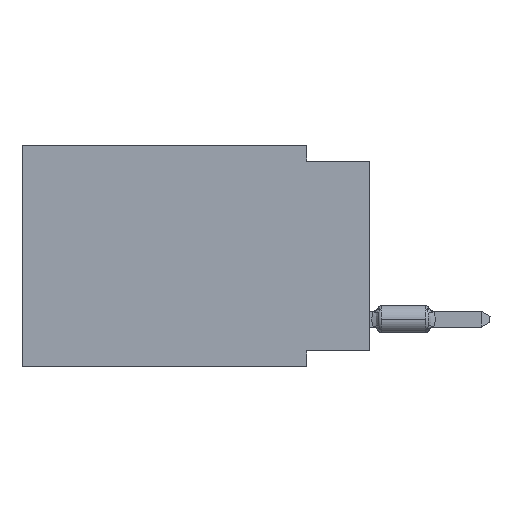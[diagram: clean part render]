
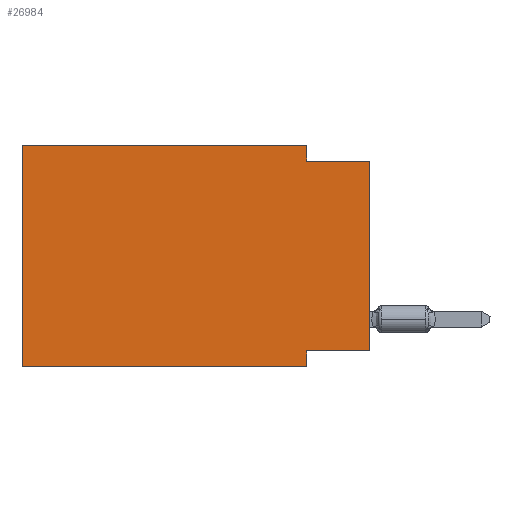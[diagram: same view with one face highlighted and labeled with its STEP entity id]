
A CAD part, left-side view. The second image highlights one B-rep face of the part: STEP entity #26984.
In plain terms, the highlighted planar face has unit normal (-1, 0, 0).
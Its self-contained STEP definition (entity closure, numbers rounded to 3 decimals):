
#285 = CARTESIAN_POINT ( 'NONE',  ( 0., 0., 0. ) ) ;
#792 = EDGE_CURVE ( 'NONE', #8059, #13492, #8434, .T. ) ;
#1193 = CARTESIAN_POINT ( 'NONE',  ( 0., 13.97, 0. ) ) ;
#1376 = LINE ( 'NONE', #13339, #2917 ) ;
#1518 = DIRECTION ( 'NONE',  ( 0., 0., -1. ) ) ;
#1552 = EDGE_CURVE ( 'NONE', #6276, #4184, #1376, .T. ) ;
#1612 = VECTOR ( 'NONE', #5593, 1000. ) ;
#1781 = ORIENTED_EDGE ( 'NONE', *, *, #23524, .F. ) ;
#2917 = VECTOR ( 'NONE', #1518, 1000. ) ;
#2962 = CARTESIAN_POINT ( 'NONE',  ( 0., 13.97, 0. ) ) ;
#3101 = ORIENTED_EDGE ( 'NONE', *, *, #22007, .F. ) ;
#3314 = VECTOR ( 'NONE', #18059, 1000. ) ;
#3389 = VERTEX_POINT ( 'NONE', #10796 ) ;
#4184 = VERTEX_POINT ( 'NONE', #19512 ) ;
#4449 = ORIENTED_EDGE ( 'NONE', *, *, #1552, .F. ) ;
#4473 = CARTESIAN_POINT ( 'NONE',  ( 0., 2.54, -0.635 ) ) ;
#5593 = DIRECTION ( 'NONE',  ( 0., 0., 1. ) ) ;
#6276 = VERTEX_POINT ( 'NONE', #9150 ) ;
#6960 = CARTESIAN_POINT ( 'NONE',  ( 0., 13.97, 0. ) ) ;
#7283 = VERTEX_POINT ( 'NONE', #8411 ) ;
#8059 = VERTEX_POINT ( 'NONE', #15459 ) ;
#8139 = ORIENTED_EDGE ( 'NONE', *, *, #12752, .T. ) ;
#8185 = DIRECTION ( 'NONE',  ( 1., 0., 0. ) ) ;
#8411 = CARTESIAN_POINT ( 'NONE',  ( 0., 13.97, -8.89 ) ) ;
#8434 = LINE ( 'NONE', #25075, #18988 ) ;
#8496 = LINE ( 'NONE', #19841, #26271 ) ;
#8830 = VECTOR ( 'NONE', #25427, 1000. ) ;
#9150 = CARTESIAN_POINT ( 'NONE',  ( 0., 2.54, -8.255 ) ) ;
#10796 = CARTESIAN_POINT ( 'NONE',  ( 0., 0., -0.635 ) ) ;
#10945 = LINE ( 'NONE', #20326, #3314 ) ;
#11613 = LINE ( 'NONE', #18587, #22914 ) ;
#12541 = ORIENTED_EDGE ( 'NONE', *, *, #29411, .F. ) ;
#12752 = EDGE_CURVE ( 'NONE', #17000, #3389, #23470, .T. ) ;
#13339 = CARTESIAN_POINT ( 'NONE',  ( 0., 2.54, -8.89 ) ) ;
#13492 = VERTEX_POINT ( 'NONE', #4473 ) ;
#13891 = CARTESIAN_POINT ( 'NONE',  ( 0., 0., -8.255 ) ) ;
#15459 = CARTESIAN_POINT ( 'NONE',  ( 0., 2.54, 0. ) ) ;
#17000 = VERTEX_POINT ( 'NONE', #13891 ) ;
#17668 = DIRECTION ( 'NONE',  ( 0., 0., -1. ) ) ;
#18000 = DIRECTION ( 'NONE',  ( 0., 1., 0. ) ) ;
#18059 = DIRECTION ( 'NONE',  ( 0., -1., 0. ) ) ;
#18424 = DIRECTION ( 'NONE',  ( 0., -1., 0. ) ) ;
#18587 = CARTESIAN_POINT ( 'NONE',  ( 0., 0., -0.635 ) ) ;
#18988 = VECTOR ( 'NONE', #17668, 1000. ) ;
#19512 = CARTESIAN_POINT ( 'NONE',  ( 0., 2.54, -8.89 ) ) ;
#19550 = DIRECTION ( 'NONE',  ( 0., -1., 0. ) ) ;
#19697 = AXIS2_PLACEMENT_3D ( 'NONE', #1193, #8185, #26635 ) ;
#19841 = CARTESIAN_POINT ( 'NONE',  ( 0., 13.97, -8.89 ) ) ;
#20326 = CARTESIAN_POINT ( 'NONE',  ( 0., 13.97, 0. ) ) ;
#20577 = LINE ( 'NONE', #22699, #23340 ) ;
#20653 = EDGE_CURVE ( 'NONE', #7283, #4184, #8496, .T. ) ;
#21881 = EDGE_CURVE ( 'NONE', #17000, #6276, #20577, .T. ) ;
#21961 = PLANE ( 'NONE',  #19697 ) ;
#22007 = EDGE_CURVE ( 'NONE', #7283, #28661, #27674, .T. ) ;
#22699 = CARTESIAN_POINT ( 'NONE',  ( 0., 0., -8.255 ) ) ;
#22914 = VECTOR ( 'NONE', #18424, 1000. ) ;
#23340 = VECTOR ( 'NONE', #18000, 1000. ) ;
#23470 = LINE ( 'NONE', #285, #1612 ) ;
#23524 = EDGE_CURVE ( 'NONE', #13492, #3389, #11613, .T. ) ;
#24394 = ORIENTED_EDGE ( 'NONE', *, *, #21881, .F. ) ;
#24813 = FACE_OUTER_BOUND ( 'NONE', #27168, .T. ) ;
#25075 = CARTESIAN_POINT ( 'NONE',  ( 0., 2.54, 0. ) ) ;
#25427 = DIRECTION ( 'NONE',  ( 0., 0., 1. ) ) ;
#26271 = VECTOR ( 'NONE', #19550, 1000. ) ;
#26272 = ORIENTED_EDGE ( 'NONE', *, *, #20653, .T. ) ;
#26635 = DIRECTION ( 'NONE',  ( 0., 0., -1. ) ) ;
#26984 = ADVANCED_FACE ( 'NONE', ( #24813 ), #21961, .F. ) ;
#27168 = EDGE_LOOP ( 'NONE', ( #8139, #1781, #27588, #12541, #3101, #26272, #4449, #24394 ) ) ;
#27588 = ORIENTED_EDGE ( 'NONE', *, *, #792, .F. ) ;
#27674 = LINE ( 'NONE', #6960, #8830 ) ;
#28661 = VERTEX_POINT ( 'NONE', #2962 ) ;
#29411 = EDGE_CURVE ( 'NONE', #28661, #8059, #10945, .T. ) ;
